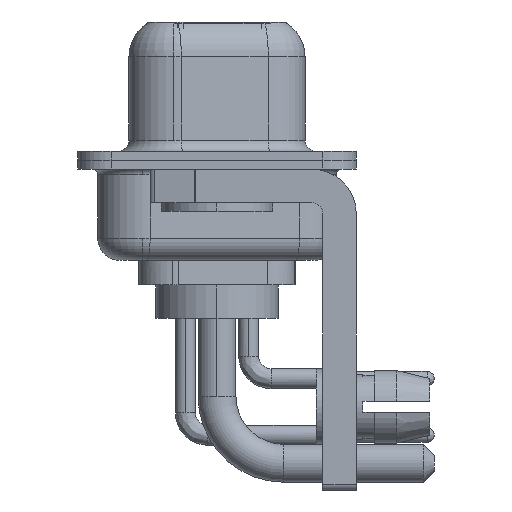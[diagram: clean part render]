
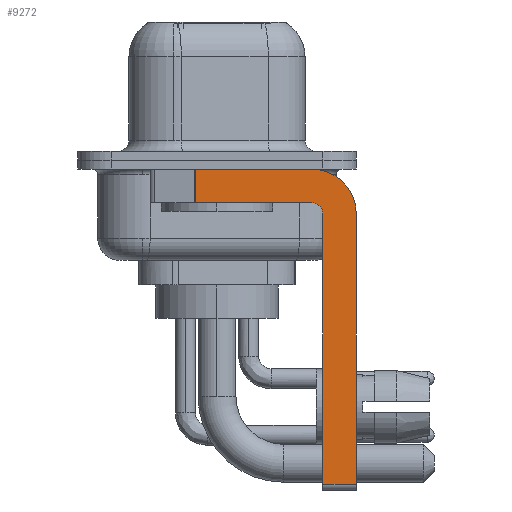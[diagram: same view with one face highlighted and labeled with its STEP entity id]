
A CAD part, left-side view. The second image highlights one B-rep face of the part: STEP entity #9272.
In plain terms, the highlighted planar face has unit normal (-1, 0, 0).
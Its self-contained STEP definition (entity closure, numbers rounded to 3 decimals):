
#252 = ORIENTED_EDGE ( 'NONE', *, *, #7851, .F. ) ;
#657 = EDGE_LOOP ( 'NONE', ( #14390, #13329, #20276, #252, #2176, #14188, #9289, #2350 ) ) ;
#749 = CARTESIAN_POINT ( 'NONE',  ( -2.9, -6.25, -2.4 ) ) ;
#763 = EDGE_CURVE ( 'NONE', #4705, #13552, #9194, .T. ) ;
#810 = CARTESIAN_POINT ( 'NONE',  ( -2.9, -4.25, -2.4 ) ) ;
#2039 = DIRECTION ( 'NONE',  ( 0., 0., -1. ) ) ;
#2081 = VERTEX_POINT ( 'NONE', #17976 ) ;
#2097 = VECTOR ( 'NONE', #18710, 1000. ) ;
#2176 = ORIENTED_EDGE ( 'NONE', *, *, #17866, .F. ) ;
#2264 = VERTEX_POINT ( 'NONE', #11806 ) ;
#2350 = ORIENTED_EDGE ( 'NONE', *, *, #8959, .F. ) ;
#4542 = CARTESIAN_POINT ( 'NONE',  ( -2.9, 0.978, -1.9 ) ) ;
#4705 = VERTEX_POINT ( 'NONE', #13564 ) ;
#5908 = EDGE_CURVE ( 'NONE', #10709, #16562, #9699, .T. ) ;
#6053 = DIRECTION ( 'NONE',  ( 0., 0., -1. ) ) ;
#6148 = CARTESIAN_POINT ( 'NONE',  ( -2.9, -4.25, -1.9 ) ) ;
#6328 = CARTESIAN_POINT ( 'NONE',  ( -2.9, 0.978, -1.9 ) ) ;
#6329 = VERTEX_POINT ( 'NONE', #7605 ) ;
#6619 = CIRCLE ( 'NONE', #11004, 0.5 ) ;
#6688 = CARTESIAN_POINT ( 'NONE',  ( -2.9, -4.25, -14.55 ) ) ;
#7059 = FACE_OUTER_BOUND ( 'NONE', #657, .T. ) ;
#7105 = EDGE_CURVE ( 'NONE', #2081, #13552, #12170, .T. ) ;
#7170 = DIRECTION ( 'NONE',  ( 1., 0., 0. ) ) ;
#7258 = LINE ( 'NONE', #19502, #12654 ) ;
#7605 = CARTESIAN_POINT ( 'NONE',  ( -2.9, -4.75, -2.4 ) ) ;
#7851 = EDGE_CURVE ( 'NONE', #6329, #10709, #6619, .T. ) ;
#8959 = EDGE_CURVE ( 'NONE', #16486, #4705, #18738, .T. ) ;
#9194 = LINE ( 'NONE', #749, #19245 ) ;
#9241 = AXIS2_PLACEMENT_3D ( 'NONE', #12219, #7170, #2039 ) ;
#9272 = ADVANCED_FACE ( 'NONE', ( #7059 ), #19522, .F. ) ;
#9289 = ORIENTED_EDGE ( 'NONE', *, *, #763, .F. ) ;
#9699 = LINE ( 'NONE', #6148, #18986 ) ;
#9971 = AXIS2_PLACEMENT_3D ( 'NONE', #810, #14309, #6053 ) ;
#10709 = VERTEX_POINT ( 'NONE', #21029 ) ;
#11004 = AXIS2_PLACEMENT_3D ( 'NONE', #11661, #18634, #13475 ) ;
#11661 = CARTESIAN_POINT ( 'NONE',  ( -2.9, -4.25, -2.4 ) ) ;
#11714 = CARTESIAN_POINT ( 'NONE',  ( -2.9, -4.25, -0.4 ) ) ;
#11806 = CARTESIAN_POINT ( 'NONE',  ( -2.9, 0.978, -0.4 ) ) ;
#12170 = LINE ( 'NONE', #6688, #18290 ) ;
#12219 = CARTESIAN_POINT ( 'NONE',  ( -2.9, -4.25, -2.4 ) ) ;
#12585 = CARTESIAN_POINT ( 'NONE',  ( -2.9, -6.25, -14.55 ) ) ;
#12654 = VECTOR ( 'NONE', #12747, 1000. ) ;
#12747 = DIRECTION ( 'NONE',  ( 0., -1., 0. ) ) ;
#13123 = DIRECTION ( 'NONE',  ( 0., 1., 0. ) ) ;
#13329 = ORIENTED_EDGE ( 'NONE', *, *, #14616, .T. ) ;
#13475 = DIRECTION ( 'NONE',  ( 0., 0., 1. ) ) ;
#13552 = VERTEX_POINT ( 'NONE', #12585 ) ;
#13564 = CARTESIAN_POINT ( 'NONE',  ( -2.9, -6.25, -2.4 ) ) ;
#13678 = DIRECTION ( 'NONE',  ( 0., 0., 1. ) ) ;
#13768 = DIRECTION ( 'NONE',  ( 0., -1., 0. ) ) ;
#14188 = ORIENTED_EDGE ( 'NONE', *, *, #7105, .T. ) ;
#14309 = DIRECTION ( 'NONE',  ( 1., 0., 0. ) ) ;
#14390 = ORIENTED_EDGE ( 'NONE', *, *, #19315, .F. ) ;
#14616 = EDGE_CURVE ( 'NONE', #2264, #16562, #21907, .T. ) ;
#15931 = VECTOR ( 'NONE', #13678, 1000. ) ;
#16171 = DIRECTION ( 'NONE',  ( 0., 0., -1. ) ) ;
#16486 = VERTEX_POINT ( 'NONE', #11714 ) ;
#16562 = VERTEX_POINT ( 'NONE', #6328 ) ;
#17866 = EDGE_CURVE ( 'NONE', #2081, #6329, #18726, .T. ) ;
#17976 = CARTESIAN_POINT ( 'NONE',  ( -2.9, -4.75, -14.55 ) ) ;
#18290 = VECTOR ( 'NONE', #13768, 1000. ) ;
#18634 = DIRECTION ( 'NONE',  ( -1., 0., 0. ) ) ;
#18710 = DIRECTION ( 'NONE',  ( 0., 0., -1. ) ) ;
#18726 = LINE ( 'NONE', #22599, #15931 ) ;
#18738 = CIRCLE ( 'NONE', #9971, 2. ) ;
#18986 = VECTOR ( 'NONE', #13123, 1000. ) ;
#19245 = VECTOR ( 'NONE', #16171, 1000. ) ;
#19315 = EDGE_CURVE ( 'NONE', #2264, #16486, #7258, .T. ) ;
#19502 = CARTESIAN_POINT ( 'NONE',  ( -2.9, 3., -0.4 ) ) ;
#19522 = PLANE ( 'NONE',  #9241 ) ;
#20276 = ORIENTED_EDGE ( 'NONE', *, *, #5908, .F. ) ;
#21029 = CARTESIAN_POINT ( 'NONE',  ( -2.9, -4.25, -1.9 ) ) ;
#21907 = LINE ( 'NONE', #4542, #2097 ) ;
#22599 = CARTESIAN_POINT ( 'NONE',  ( -2.9, -4.75, -14.8 ) ) ;
